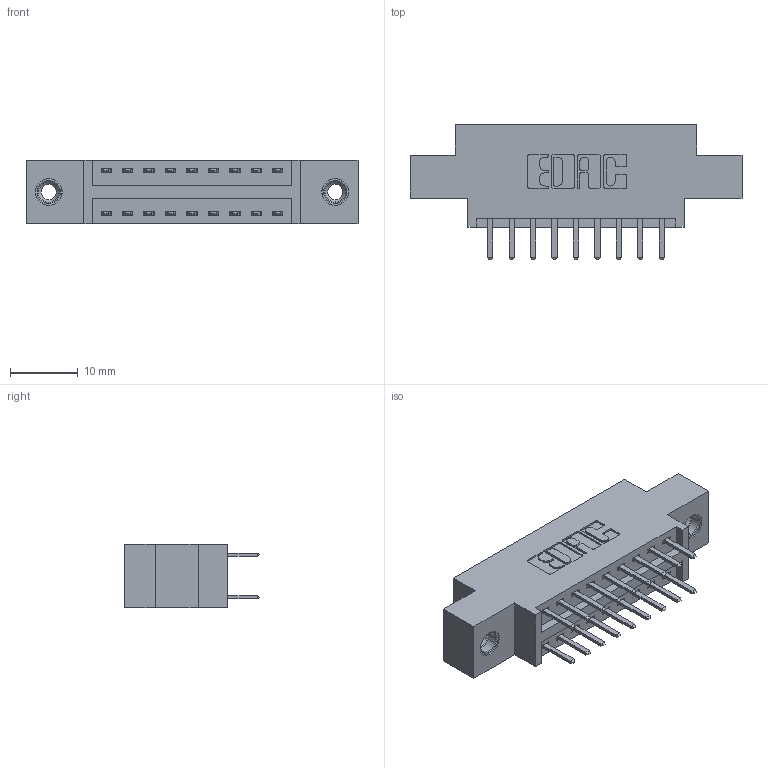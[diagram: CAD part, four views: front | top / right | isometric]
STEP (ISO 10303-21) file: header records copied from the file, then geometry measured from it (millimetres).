
FILE_DESCRIPTION (( 'STEP AP203' ), '1' );
FILE_NAME ('396-018-520-808.STEP', '2018-09-01T01:34:04', ( '' ), ( '' ), 'SwSTEP 2.0', 'SolidWorks 2016', '' );
FILE_SCHEMA (( 'CONFIG_CONTROL_DESIGN' ));
Length unit declared in the file: inch
Products named in the file (4): 346 Part_0.170 Offset - 0.156 Dia-TI; 345-292-001_345-293-120; 345-250-001_345-250-003-102; 396-018-520-808
Assembly tree (21 placements, depth 2):
  396-018-520-808
    346 Part_0.170 Offset - 0.156 Dia-TI
    345-292-001_345-293-120  x18
    345-250-001_345-250-003-102  x2
Bounding box: 49.15 x 20.02 x 9.4 mm (x, y, z)
Volume: 4367.3 mm3; surface area: 5665.6 mm2
Topology: 21 solids, 21 shells, 1194 faces, 3411 edges, 2218 vertices
Faces by surface type: plane 778, cylinder 400, cone 12, torus 4
Entity records: 11748 total; most frequent: CARTESIAN_POINT 1979, ORIENTED_EDGE 1894, DIRECTION 1809, EDGE_CURVE 947, VECTOR 755, LINE 755, VERTEX_POINT 624, AXIS2_PLACEMENT_3D 527
